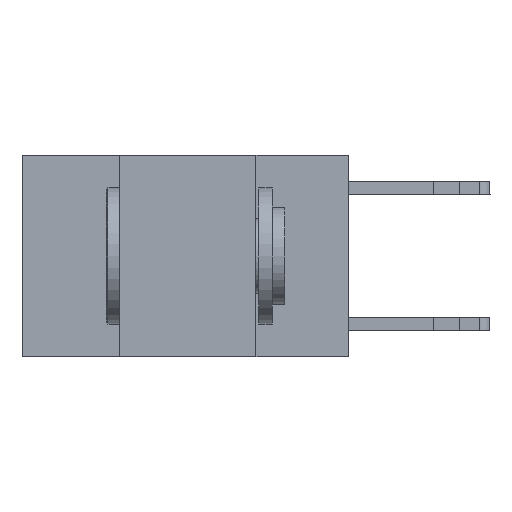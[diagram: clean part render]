
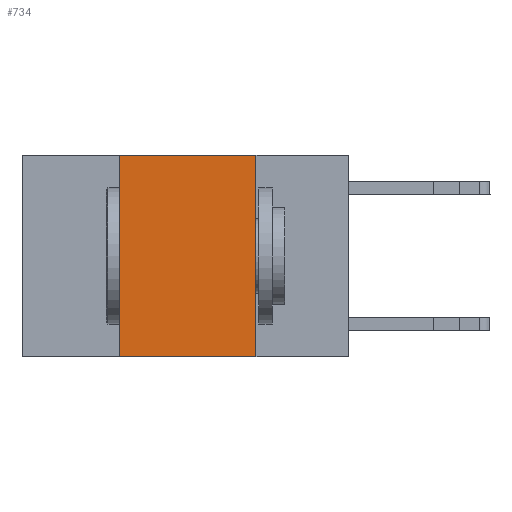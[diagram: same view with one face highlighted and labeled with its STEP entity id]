
A CAD part, left-side view. The second image highlights one B-rep face of the part: STEP entity #734.
In plain terms, the highlighted planar face has unit normal (-1, 0, 0).
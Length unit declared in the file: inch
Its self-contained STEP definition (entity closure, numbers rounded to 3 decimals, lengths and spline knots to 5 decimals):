
#245 = ORIENTED_EDGE ( 'NONE', *, *, #402, .T. ) ;
#402 = EDGE_CURVE ( 'NONE', #15807, #12039, #1538, .T. ) ;
#734 = ADVANCED_FACE ( 'NONE', ( #10802 ), #4331, .F. ) ;
#895 = CARTESIAN_POINT ( 'NONE',  ( 0., 0.17, 0. ) ) ;
#1380 = DIRECTION ( 'NONE',  ( 0., -1., 0. ) ) ;
#1422 = DIRECTION ( 'NONE',  ( 0., -1., 0. ) ) ;
#1538 = LINE ( 'NONE', #16207, #16549 ) ;
#2024 = ORIENTED_EDGE ( 'NONE', *, *, #4764, .F. ) ;
#2218 = VERTEX_POINT ( 'NONE', #895 ) ;
#2394 = DIRECTION ( 'NONE',  ( 0., 0., 1. ) ) ;
#3339 = LINE ( 'NONE', #9921, #3584 ) ;
#3584 = VECTOR ( 'NONE', #1380, 39.37008 ) ;
#3640 = DIRECTION ( 'NONE',  ( 0., 0., -1. ) ) ;
#3988 = EDGE_LOOP ( 'NONE', ( #2024, #12214, #16526, #245 ) ) ;
#4331 = PLANE ( 'NONE',  #7608 ) ;
#4764 = EDGE_CURVE ( 'NONE', #2218, #12039, #14997, .T. ) ;
#4836 = VECTOR ( 'NONE', #3640, 39.37008 ) ;
#5263 = CARTESIAN_POINT ( 'NONE',  ( 0., 0.17, 0. ) ) ;
#5313 = CARTESIAN_POINT ( 'NONE',  ( 0., 0.42, 0. ) ) ;
#7608 = AXIS2_PLACEMENT_3D ( 'NONE', #17389, #12540, #10586 ) ;
#8245 = EDGE_CURVE ( 'NONE', #14439, #2218, #3339, .T. ) ;
#9921 = CARTESIAN_POINT ( 'NONE',  ( 0., 0.6, 0. ) ) ;
#10396 = CARTESIAN_POINT ( 'NONE',  ( 0., 0.42, -0.37 ) ) ;
#10556 = CARTESIAN_POINT ( 'NONE',  ( 0., 0.42, 0. ) ) ;
#10586 = DIRECTION ( 'NONE',  ( 0., 0., -1. ) ) ;
#10802 = FACE_OUTER_BOUND ( 'NONE', #3988, .T. ) ;
#12039 = VERTEX_POINT ( 'NONE', #18385 ) ;
#12214 = ORIENTED_EDGE ( 'NONE', *, *, #8245, .F. ) ;
#12540 = DIRECTION ( 'NONE',  ( 1., 0., 0. ) ) ;
#14439 = VERTEX_POINT ( 'NONE', #10556 ) ;
#14997 = LINE ( 'NONE', #5263, #4836 ) ;
#15807 = VERTEX_POINT ( 'NONE', #10396 ) ;
#16207 = CARTESIAN_POINT ( 'NONE',  ( 0., 0.6, -0.37 ) ) ;
#16245 = EDGE_CURVE ( 'NONE', #15807, #14439, #20097, .T. ) ;
#16526 = ORIENTED_EDGE ( 'NONE', *, *, #16245, .F. ) ;
#16549 = VECTOR ( 'NONE', #1422, 39.37008 ) ;
#17323 = VECTOR ( 'NONE', #2394, 39.37008 ) ;
#17389 = CARTESIAN_POINT ( 'NONE',  ( 0., 0.6, 0. ) ) ;
#18385 = CARTESIAN_POINT ( 'NONE',  ( 0., 0.17, -0.37 ) ) ;
#20097 = LINE ( 'NONE', #5313, #17323 ) ;
